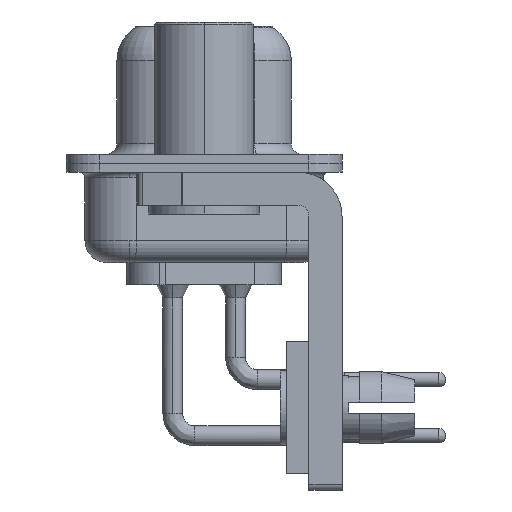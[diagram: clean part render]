
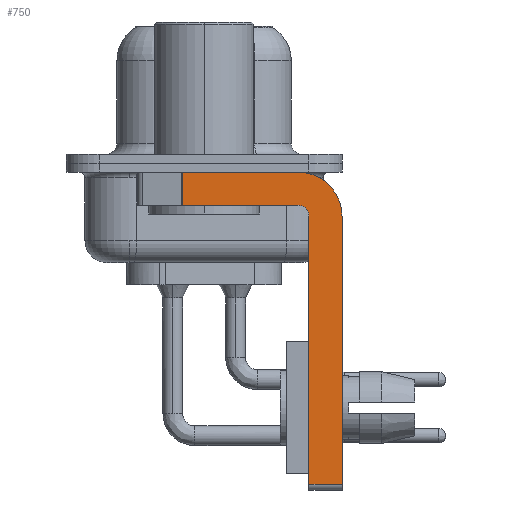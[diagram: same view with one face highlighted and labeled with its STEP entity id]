
A CAD part, left-side view. The second image highlights one B-rep face of the part: STEP entity #750.
In plain terms, the highlighted planar face has unit normal (-1, 0, 0).
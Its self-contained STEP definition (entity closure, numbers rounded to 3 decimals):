
#28 = ORIENTED_EDGE ( 'NONE', *, *, #30163, .F. ) ;
#750 = ADVANCED_FACE ( 'NONE', ( #18278 ), #28079, .F. ) ;
#1006 = EDGE_CURVE ( 'NONE', #13650, #11990, #4986, .T. ) ;
#1027 = CARTESIAN_POINT ( 'NONE',  ( -2.9, -4.25, -0.4 ) ) ;
#1521 = VECTOR ( 'NONE', #13214, 1000. ) ;
#2210 = DIRECTION ( 'NONE',  ( 0., 0., -1. ) ) ;
#3451 = EDGE_LOOP ( 'NONE', ( #28, #33022, #10327, #16746, #11038, #21696, #18403, #32486 ) ) ;
#4540 = CIRCLE ( 'NONE', #5839, 0.5 ) ;
#4903 = VECTOR ( 'NONE', #33391, 1000. ) ;
#4970 = CARTESIAN_POINT ( 'NONE',  ( -2.9, -6.25, -2.4 ) ) ;
#4986 = LINE ( 'NONE', #31647, #31576 ) ;
#5839 = AXIS2_PLACEMENT_3D ( 'NONE', #11282, #29227, #13830 ) ;
#6161 = VERTEX_POINT ( 'NONE', #8394 ) ;
#6419 = VECTOR ( 'NONE', #31750, 1000. ) ;
#7065 = DIRECTION ( 'NONE',  ( 0., 0., -1. ) ) ;
#8394 = CARTESIAN_POINT ( 'NONE',  ( -2.9, -4.75, -2.4 ) ) ;
#9144 = AXIS2_PLACEMENT_3D ( 'NONE', #10673, #28633, #13238 ) ;
#10327 = ORIENTED_EDGE ( 'NONE', *, *, #27868, .F. ) ;
#10656 = CARTESIAN_POINT ( 'NONE',  ( -2.9, -4.25, -14.55 ) ) ;
#10673 = CARTESIAN_POINT ( 'NONE',  ( -2.9, -4.25, -2.4 ) ) ;
#11038 = ORIENTED_EDGE ( 'NONE', *, *, #31742, .F. ) ;
#11094 = EDGE_CURVE ( 'NONE', #6161, #31631, #4540, .T. ) ;
#11282 = CARTESIAN_POINT ( 'NONE',  ( -2.9, -4.25, -2.4 ) ) ;
#11990 = VERTEX_POINT ( 'NONE', #22571 ) ;
#13214 = DIRECTION ( 'NONE',  ( 0., -1., 0. ) ) ;
#13238 = DIRECTION ( 'NONE',  ( 0., 0., -1. ) ) ;
#13307 = LINE ( 'NONE', #29159, #6419 ) ;
#13318 = CARTESIAN_POINT ( 'NONE',  ( -2.9, -4.25, -1.9 ) ) ;
#13496 = VERTEX_POINT ( 'NONE', #23709 ) ;
#13650 = VERTEX_POINT ( 'NONE', #14538 ) ;
#13830 = DIRECTION ( 'NONE',  ( 0., 0., 1. ) ) ;
#14538 = CARTESIAN_POINT ( 'NONE',  ( -2.9, 0.978, -0.4 ) ) ;
#16746 = ORIENTED_EDGE ( 'NONE', *, *, #11094, .F. ) ;
#17989 = DIRECTION ( 'NONE',  ( 0., -1., 0. ) ) ;
#18278 = FACE_OUTER_BOUND ( 'NONE', #3451, .T. ) ;
#18403 = ORIENTED_EDGE ( 'NONE', *, *, #28776, .F. ) ;
#18593 = LINE ( 'NONE', #4970, #4903 ) ;
#18915 = VECTOR ( 'NONE', #17989, 1000. ) ;
#19078 = EDGE_CURVE ( 'NONE', #29583, #27685, #33306, .T. ) ;
#20616 = LINE ( 'NONE', #22059, #26710 ) ;
#20656 = CARTESIAN_POINT ( 'NONE',  ( -2.9, -4.75, -14.55 ) ) ;
#21696 = ORIENTED_EDGE ( 'NONE', *, *, #25143, .T. ) ;
#22059 = CARTESIAN_POINT ( 'NONE',  ( -2.9, -4.25, -1.9 ) ) ;
#22571 = CARTESIAN_POINT ( 'NONE',  ( -2.9, 0.978, -1.9 ) ) ;
#23004 = CARTESIAN_POINT ( 'NONE',  ( -2.9, 3., -0.4 ) ) ;
#23709 = CARTESIAN_POINT ( 'NONE',  ( -2.9, -6.25, -14.55 ) ) ;
#23795 = VERTEX_POINT ( 'NONE', #20656 ) ;
#23910 = CARTESIAN_POINT ( 'NONE',  ( -2.9, -6.25, -2.4 ) ) ;
#25143 = EDGE_CURVE ( 'NONE', #23795, #13496, #28935, .T. ) ;
#25750 = LINE ( 'NONE', #23004, #18915 ) ;
#26710 = VECTOR ( 'NONE', #27308, 1000. ) ;
#27308 = DIRECTION ( 'NONE',  ( 0., 1., 0. ) ) ;
#27366 = DIRECTION ( 'NONE',  ( 1., 0., 0. ) ) ;
#27685 = VERTEX_POINT ( 'NONE', #23910 ) ;
#27868 = EDGE_CURVE ( 'NONE', #31631, #11990, #20616, .T. ) ;
#28079 = PLANE ( 'NONE',  #31344 ) ;
#28221 = CARTESIAN_POINT ( 'NONE',  ( -2.9, -4.25, -2.4 ) ) ;
#28633 = DIRECTION ( 'NONE',  ( 1., 0., 0. ) ) ;
#28776 = EDGE_CURVE ( 'NONE', #27685, #13496, #18593, .T. ) ;
#28935 = LINE ( 'NONE', #10656, #1521 ) ;
#29159 = CARTESIAN_POINT ( 'NONE',  ( -2.9, -4.75, -14.8 ) ) ;
#29227 = DIRECTION ( 'NONE',  ( -1., 0., 0. ) ) ;
#29583 = VERTEX_POINT ( 'NONE', #1027 ) ;
#30163 = EDGE_CURVE ( 'NONE', #13650, #29583, #25750, .T. ) ;
#31344 = AXIS2_PLACEMENT_3D ( 'NONE', #28221, #27366, #2210 ) ;
#31576 = VECTOR ( 'NONE', #7065, 1000. ) ;
#31631 = VERTEX_POINT ( 'NONE', #13318 ) ;
#31647 = CARTESIAN_POINT ( 'NONE',  ( -2.9, 0.978, -1.9 ) ) ;
#31742 = EDGE_CURVE ( 'NONE', #23795, #6161, #13307, .T. ) ;
#31750 = DIRECTION ( 'NONE',  ( 0., 0., 1. ) ) ;
#32486 = ORIENTED_EDGE ( 'NONE', *, *, #19078, .F. ) ;
#33022 = ORIENTED_EDGE ( 'NONE', *, *, #1006, .T. ) ;
#33306 = CIRCLE ( 'NONE', #9144, 2. ) ;
#33391 = DIRECTION ( 'NONE',  ( 0., 0., -1. ) ) ;
